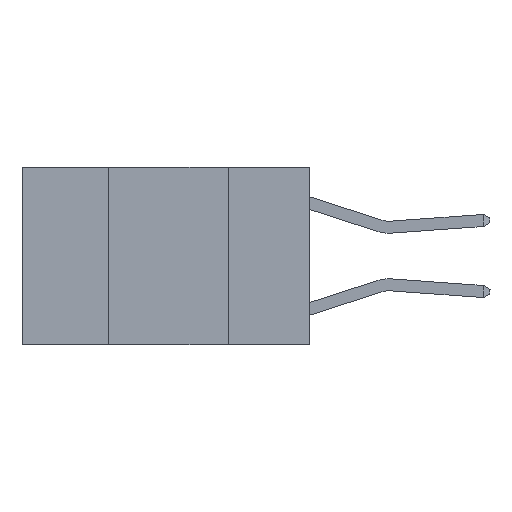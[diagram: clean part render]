
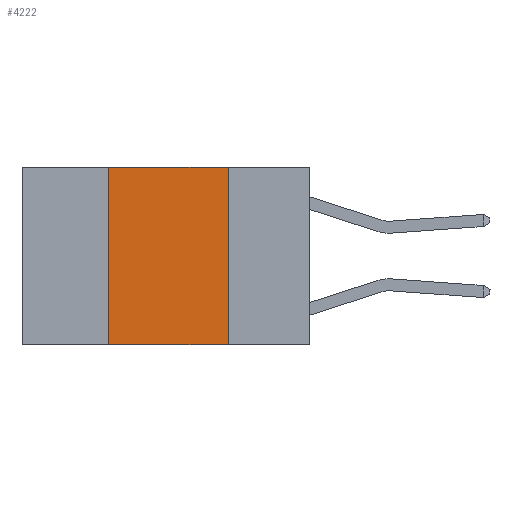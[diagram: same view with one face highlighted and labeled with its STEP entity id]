
A CAD part, left-side view. The second image highlights one B-rep face of the part: STEP entity #4222.
In plain terms, the highlighted planar face has unit normal (-1, 0, 0).
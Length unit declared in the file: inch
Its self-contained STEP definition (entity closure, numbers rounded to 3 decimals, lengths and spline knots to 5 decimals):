
#2377 = CARTESIAN_POINT ( 'NONE',  ( 0., 0.42, 0. ) ) ;
#2948 = EDGE_LOOP ( 'NONE', ( #23030, #7611, #4092, #14928 ) ) ;
#3478 = DIRECTION ( 'NONE',  ( 0., 0., -1. ) ) ;
#4092 = ORIENTED_EDGE ( 'NONE', *, *, #5612, .F. ) ;
#4189 = CARTESIAN_POINT ( 'NONE',  ( 0., 0.17, 0. ) ) ;
#4222 = ADVANCED_FACE ( 'NONE', ( #18575 ), #13652, .F. ) ;
#4240 = EDGE_CURVE ( 'NONE', #19332, #12727, #13252, .T. ) ;
#4488 = VERTEX_POINT ( 'NONE', #4189 ) ;
#5612 = EDGE_CURVE ( 'NONE', #19332, #11276, #9357, .T. ) ;
#6308 = DIRECTION ( 'NONE',  ( 0., 0., 1. ) ) ;
#6997 = EDGE_CURVE ( 'NONE', #4488, #12727, #15672, .T. ) ;
#7611 = ORIENTED_EDGE ( 'NONE', *, *, #21736, .F. ) ;
#8738 = CARTESIAN_POINT ( 'NONE',  ( 0., 0.17, 0. ) ) ;
#9034 = CARTESIAN_POINT ( 'NONE',  ( 0., 0.17, -0.37 ) ) ;
#9357 = LINE ( 'NONE', #20075, #19451 ) ;
#9565 = CARTESIAN_POINT ( 'NONE',  ( 0., 0.6, 0. ) ) ;
#9739 = VECTOR ( 'NONE', #12006, 39.37008 ) ;
#9944 = CARTESIAN_POINT ( 'NONE',  ( 0., 0.6, 0. ) ) ;
#10812 = DIRECTION ( 'NONE',  ( 0., 0., -1. ) ) ;
#11276 = VERTEX_POINT ( 'NONE', #2377 ) ;
#11714 = CARTESIAN_POINT ( 'NONE',  ( 0., 0.6, -0.37 ) ) ;
#12006 = DIRECTION ( 'NONE',  ( 0., -1., 0. ) ) ;
#12638 = VECTOR ( 'NONE', #13741, 39.37008 ) ;
#12727 = VERTEX_POINT ( 'NONE', #9034 ) ;
#13252 = LINE ( 'NONE', #11714, #12638 ) ;
#13652 = PLANE ( 'NONE',  #20979 ) ;
#13741 = DIRECTION ( 'NONE',  ( 0., -1., 0. ) ) ;
#14928 = ORIENTED_EDGE ( 'NONE', *, *, #4240, .T. ) ;
#15131 = LINE ( 'NONE', #9944, #9739 ) ;
#15672 = LINE ( 'NONE', #8738, #19729 ) ;
#15675 = DIRECTION ( 'NONE',  ( 1., 0., 0. ) ) ;
#18575 = FACE_OUTER_BOUND ( 'NONE', #2948, .T. ) ;
#19332 = VERTEX_POINT ( 'NONE', #21844 ) ;
#19451 = VECTOR ( 'NONE', #6308, 39.37008 ) ;
#19729 = VECTOR ( 'NONE', #10812, 39.37008 ) ;
#20075 = CARTESIAN_POINT ( 'NONE',  ( 0., 0.42, 0. ) ) ;
#20979 = AXIS2_PLACEMENT_3D ( 'NONE', #9565, #15675, #3478 ) ;
#21736 = EDGE_CURVE ( 'NONE', #11276, #4488, #15131, .T. ) ;
#21844 = CARTESIAN_POINT ( 'NONE',  ( 0., 0.42, -0.37 ) ) ;
#23030 = ORIENTED_EDGE ( 'NONE', *, *, #6997, .F. ) ;
